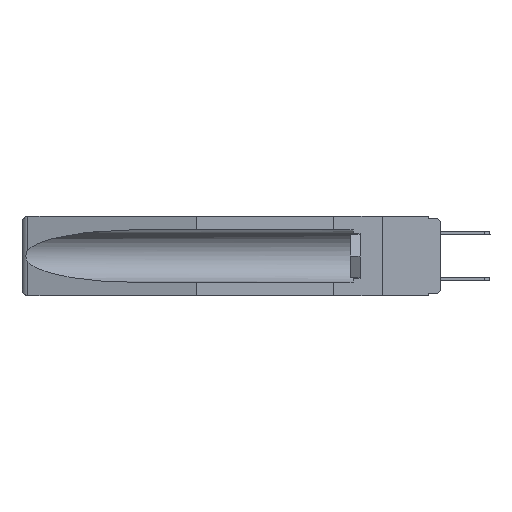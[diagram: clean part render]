
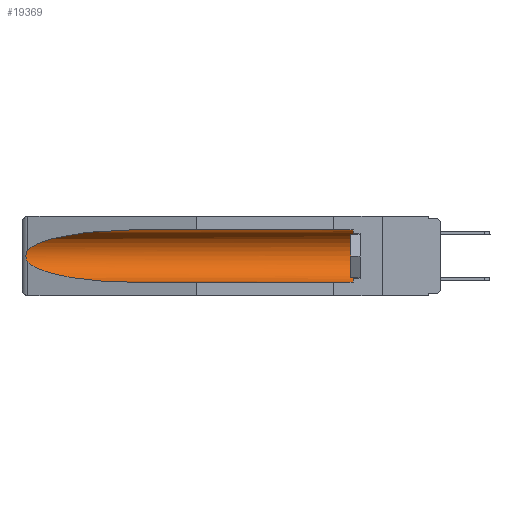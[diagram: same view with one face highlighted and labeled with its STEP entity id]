
A CAD part, left-side view. The second image highlights one B-rep face of the part: STEP entity #19369.
In plain terms, the highlighted cylindrical face has radius 2.857 mm (diameter 5.715 mm), a partial arc.
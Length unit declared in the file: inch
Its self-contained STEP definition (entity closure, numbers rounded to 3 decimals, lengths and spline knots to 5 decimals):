
#5 = AXIS2_PLACEMENT_3D ( 'NONE', #21251, #1734, #6619 ) ;
#173 = CARTESIAN_POINT ( 'NONE',  ( 0.26537, 1.52718, -0.19328 ) ) ;
#223 = DIRECTION ( 'NONE',  ( 0., 1., 0. ) ) ;
#1140 = ORIENTED_EDGE ( 'NONE', *, *, #16175, .T. ) ;
#1302 = CARTESIAN_POINT ( 'NONE',  ( 0.26655, 1.53094, -0.18657 ) ) ;
#1311 = AXIS2_PLACEMENT_3D ( 'NONE', #7936, #12714, #4479 ) ;
#1734 = DIRECTION ( 'NONE',  ( 0., -1., 0. ) ) ;
#3058 = LINE ( 'NONE', #13123, #4481 ) ;
#4479 = DIRECTION ( 'NONE',  ( 0., 0., 1. ) ) ;
#4481 = VECTOR ( 'NONE', #223, 39.37008 ) ;
#4553 = B_SPLINE_CURVE_WITH_KNOTS ( 'NONE', 3,
 ( #9849, #16599, #16163, #16483, #8216, #14861, #4973, #1302, #7911, #20479 ),
 .UNSPECIFIED., .F., .F.,
 ( 4, 2, 2, 2, 4 ),
 ( 0., 0.00029, 0.00058, 0.00087, 0.00117 ),
 .UNSPECIFIED. ) ;
#4973 = CARTESIAN_POINT ( 'NONE',  ( 0.2673, 1.53269, -0.17917 ) ) ;
#5351 = CARTESIAN_POINT ( 'NONE',  ( 0.25451, 1.48313, -0.24835 ) ) ;
#6095 = FACE_OUTER_BOUND ( 'NONE', #6295, .T. ) ;
#6295 = EDGE_LOOP ( 'NONE', ( #6360, #20140, #20203, #11994, #7305, #1140 ) ) ;
#6360 = ORIENTED_EDGE ( 'NONE', *, *, #10445, .T. ) ;
#6619 = DIRECTION ( 'NONE',  ( 0., 0., 1. ) ) ;
#6646 = CARTESIAN_POINT ( 'NONE',  ( 0.155, 0.126, -0.059 ) ) ;
#7123 =( BOUNDED_CURVE ( )  B_SPLINE_CURVE ( 3, ( #15885, #12282, #7520, #20750 ),
 .UNSPECIFIED., .F., .F. ) 
 B_SPLINE_CURVE_WITH_KNOTS ( ( 4, 4 ),
 ( 4.71239, 6.08839 ),
 .UNSPECIFIED. ) 
 CURVE ( )  GEOMETRIC_REPRESENTATION_ITEM ( )  RATIONAL_B_SPLINE_CURVE ( ( 1., 0.848, 0.848, 1. ) ) 
 REPRESENTATION_ITEM ( '' )  );
#7305 = ORIENTED_EDGE ( 'NONE', *, *, #14733, .T. ) ;
#7520 = CARTESIAN_POINT ( 'NONE',  ( 0.25451, 1.48313, -0.09465 ) ) ;
#7845 = VERTEX_POINT ( 'NONE', #8126 ) ;
#7911 = CARTESIAN_POINT ( 'NONE',  ( 0.26597, 1.5296, -0.19026 ) ) ;
#7936 = CARTESIAN_POINT ( 'NONE',  ( 0.155, -0.30754, -0.1715 ) ) ;
#8126 = CARTESIAN_POINT ( 'NONE',  ( 0.26537, 1.52718, -0.14972 ) ) ;
#8216 = CARTESIAN_POINT ( 'NONE',  ( 0.2675, 1.53308, -0.16763 ) ) ;
#8300 = CARTESIAN_POINT ( 'NONE',  ( 0.155, 0.126, -0.284 ) ) ;
#8517 = VECTOR ( 'NONE', #21230, 39.37008 ) ;
#8816 = VERTEX_POINT ( 'NONE', #8300 ) ;
#9614 = EDGE_CURVE ( 'NONE', #8816, #19414, #21128, .T. ) ;
#9849 = CARTESIAN_POINT ( 'NONE',  ( 0.26537, 1.52718, -0.14972 ) ) ;
#10230 = CARTESIAN_POINT ( 'NONE',  ( 0.21114, 1.30732, -0.284 ) ) ;
#10445 = EDGE_CURVE ( 'NONE', #15124, #7845, #7123, .T. ) ;
#11551 =( BOUNDED_CURVE ( )  B_SPLINE_CURVE ( 3, ( #173, #5351, #10230, #13386 ),
 .UNSPECIFIED., .F., .F. ) 
 B_SPLINE_CURVE_WITH_KNOTS ( ( 4, 4 ),
 ( 0.1948, 1.5708 ),
 .UNSPECIFIED. ) 
 CURVE ( )  GEOMETRIC_REPRESENTATION_ITEM ( )  RATIONAL_B_SPLINE_CURVE ( ( 1., 0.848, 0.848, 1. ) ) 
 REPRESENTATION_ITEM ( '' )  );
#11659 = EDGE_CURVE ( 'NONE', #15863, #19414, #11551, .T. ) ;
#11994 = ORIENTED_EDGE ( 'NONE', *, *, #9614, .F. ) ;
#12282 = CARTESIAN_POINT ( 'NONE',  ( 0.21114, 1.30732, -0.059 ) ) ;
#12714 = DIRECTION ( 'NONE',  ( 0., 1., 0. ) ) ;
#13123 = CARTESIAN_POINT ( 'NONE',  ( 0.155, -0.30754, -0.059 ) ) ;
#13279 = CARTESIAN_POINT ( 'NONE',  ( 0.26537, 1.52718, -0.19328 ) ) ;
#13386 = CARTESIAN_POINT ( 'NONE',  ( 0.155, 1.07973, -0.284 ) ) ;
#14733 = EDGE_CURVE ( 'NONE', #8816, #17511, #15939, .T. ) ;
#14861 = CARTESIAN_POINT ( 'NONE',  ( 0.2675, 1.53308, -0.17534 ) ) ;
#15124 = VERTEX_POINT ( 'NONE', #20910 ) ;
#15863 = VERTEX_POINT ( 'NONE', #13279 ) ;
#15885 = CARTESIAN_POINT ( 'NONE',  ( 0.155, 1.07973, -0.059 ) ) ;
#15939 = CIRCLE ( 'NONE', #5, 0.1125 ) ;
#16163 = CARTESIAN_POINT ( 'NONE',  ( 0.26654, 1.53092, -0.15636 ) ) ;
#16175 = EDGE_CURVE ( 'NONE', #17511, #15124, #3058, .T. ) ;
#16308 = CARTESIAN_POINT ( 'NONE',  ( 0.155, 1.07973, -0.284 ) ) ;
#16468 = CARTESIAN_POINT ( 'NONE',  ( 0.155, -0.30754, -0.284 ) ) ;
#16483 = CARTESIAN_POINT ( 'NONE',  ( 0.2673, 1.5327, -0.16383 ) ) ;
#16599 = CARTESIAN_POINT ( 'NONE',  ( 0.26597, 1.52961, -0.15275 ) ) ;
#17511 = VERTEX_POINT ( 'NONE', #6646 ) ;
#17719 = CYLINDRICAL_SURFACE ( 'NONE', #1311, 0.1125 ) ;
#18616 = EDGE_CURVE ( 'NONE', #7845, #15863, #4553, .T. ) ;
#19369 = ADVANCED_FACE ( 'NONE', ( #6095 ), #17719, .F. ) ;
#19414 = VERTEX_POINT ( 'NONE', #16308 ) ;
#20140 = ORIENTED_EDGE ( 'NONE', *, *, #18616, .T. ) ;
#20203 = ORIENTED_EDGE ( 'NONE', *, *, #11659, .T. ) ;
#20479 = CARTESIAN_POINT ( 'NONE',  ( 0.26537, 1.52718, -0.19328 ) ) ;
#20750 = CARTESIAN_POINT ( 'NONE',  ( 0.26537, 1.52718, -0.14972 ) ) ;
#20910 = CARTESIAN_POINT ( 'NONE',  ( 0.155, 1.07973, -0.059 ) ) ;
#21128 = LINE ( 'NONE', #16468, #8517 ) ;
#21230 = DIRECTION ( 'NONE',  ( 0., 1., 0. ) ) ;
#21251 = CARTESIAN_POINT ( 'NONE',  ( 0.155, 0.126, -0.1715 ) ) ;
